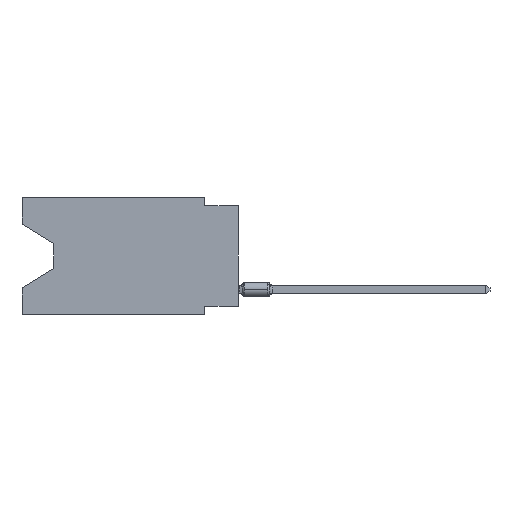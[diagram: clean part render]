
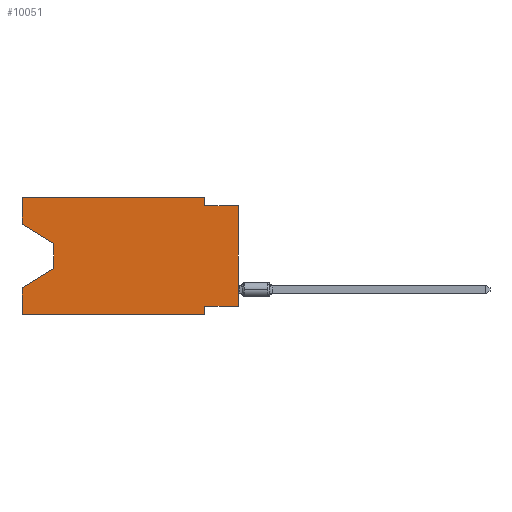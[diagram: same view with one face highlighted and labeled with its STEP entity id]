
A CAD part, left-side view. The second image highlights one B-rep face of the part: STEP entity #10051.
In plain terms, the highlighted planar face has unit normal (-1, 0, 0).
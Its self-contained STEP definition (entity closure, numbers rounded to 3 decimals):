
#285 = VERTEX_POINT ( 'NONE', #27186 ) ;
#914 = EDGE_CURVE ( 'NONE', #20251, #285, #4127, .T. ) ;
#1156 = EDGE_CURVE ( 'NONE', #26444, #12205, #14999, .T. ) ;
#1359 = ORIENTED_EDGE ( 'NONE', *, *, #14891, .F. ) ;
#1367 = CARTESIAN_POINT ( 'NONE',  ( 0., 0., -8.255 ) ) ;
#1900 = LINE ( 'NONE', #19036, #32785 ) ;
#2219 = DIRECTION ( 'NONE',  ( 0., 0.855, -0.519 ) ) ;
#2272 = VERTEX_POINT ( 'NONE', #8309 ) ;
#2441 = EDGE_CURVE ( 'NONE', #15579, #12205, #24383, .T. ) ;
#2508 = VERTEX_POINT ( 'NONE', #16016 ) ;
#3101 = VECTOR ( 'NONE', #3496, 1000. ) ;
#3142 = LINE ( 'NONE', #5683, #3101 ) ;
#3309 = DIRECTION ( 'NONE',  ( 1., 0., 0. ) ) ;
#3443 = VECTOR ( 'NONE', #9934, 1000. ) ;
#3496 = DIRECTION ( 'NONE',  ( 0., 0., 1. ) ) ;
#4127 = LINE ( 'NONE', #6864, #36004 ) ;
#4473 = DIRECTION ( 'NONE',  ( 0., -0.855, -0.519 ) ) ;
#4823 = VECTOR ( 'NONE', #21709, 1000. ) ;
#5070 = EDGE_LOOP ( 'NONE', ( #5786, #25630, #13512, #14981, #6533, #34944, #1359, #22528, #35115, #5859, #28084, #8815 ) ) ;
#5099 = VERTEX_POINT ( 'NONE', #5734 ) ;
#5683 = CARTESIAN_POINT ( 'NONE',  ( 0., 16.383, 0. ) ) ;
#5734 = CARTESIAN_POINT ( 'NONE',  ( 0., 16.383, -6.852 ) ) ;
#5786 = ORIENTED_EDGE ( 'NONE', *, *, #914, .T. ) ;
#5859 = ORIENTED_EDGE ( 'NONE', *, *, #7292, .F. ) ;
#5867 = PLANE ( 'NONE',  #7014 ) ;
#6010 = CARTESIAN_POINT ( 'NONE',  ( 0., 16.383, -8.89 ) ) ;
#6533 = ORIENTED_EDGE ( 'NONE', *, *, #31636, .T. ) ;
#6864 = CARTESIAN_POINT ( 'NONE',  ( 0., 16.383, -2.038 ) ) ;
#6902 = VECTOR ( 'NONE', #27831, 1000. ) ;
#7014 = AXIS2_PLACEMENT_3D ( 'NONE', #23020, #3309, #33968 ) ;
#7076 = CARTESIAN_POINT ( 'NONE',  ( 0., 13.97, -3.505 ) ) ;
#7292 = EDGE_CURVE ( 'NONE', #34059, #15579, #24285, .T. ) ;
#8011 = CARTESIAN_POINT ( 'NONE',  ( 0., 16.383, -8.89 ) ) ;
#8207 = VERTEX_POINT ( 'NONE', #30548 ) ;
#8309 = CARTESIAN_POINT ( 'NONE',  ( 0., 2.54, -8.89 ) ) ;
#8815 = ORIENTED_EDGE ( 'NONE', *, *, #31405, .F. ) ;
#9934 = DIRECTION ( 'NONE',  ( 0., 1., 0. ) ) ;
#9997 = LINE ( 'NONE', #7076, #15230 ) ;
#10051 = ADVANCED_FACE ( 'NONE', ( #17003 ), #5867, .F. ) ;
#10300 = DIRECTION ( 'NONE',  ( 0., 0., 1. ) ) ;
#11858 = VECTOR ( 'NONE', #2219, 1000. ) ;
#12205 = VERTEX_POINT ( 'NONE', #23962 ) ;
#13457 = DIRECTION ( 'NONE',  ( 0., -1., 0. ) ) ;
#13499 = LINE ( 'NONE', #8011, #4823 ) ;
#13512 = ORIENTED_EDGE ( 'NONE', *, *, #31322, .T. ) ;
#14691 = EDGE_CURVE ( 'NONE', #28630, #34059, #16705, .T. ) ;
#14891 = EDGE_CURVE ( 'NONE', #26444, #2508, #26363, .T. ) ;
#14909 = DIRECTION ( 'NONE',  ( 0., 0., -1. ) ) ;
#14981 = ORIENTED_EDGE ( 'NONE', *, *, #30806, .F. ) ;
#14999 = LINE ( 'NONE', #23205, #31960 ) ;
#15230 = VECTOR ( 'NONE', #23147, 1000. ) ;
#15334 = VECTOR ( 'NONE', #13457, 1000. ) ;
#15579 = VERTEX_POINT ( 'NONE', #20095 ) ;
#16016 = CARTESIAN_POINT ( 'NONE',  ( 0., 2.54, -8.255 ) ) ;
#16101 = CARTESIAN_POINT ( 'NONE',  ( 0., 16.383, 0. ) ) ;
#16273 = CARTESIAN_POINT ( 'NONE',  ( 0., 13.97, -5.385 ) ) ;
#16705 = LINE ( 'NONE', #32946, #6902 ) ;
#17003 = FACE_OUTER_BOUND ( 'NONE', #5070, .T. ) ;
#17646 = CARTESIAN_POINT ( 'NONE',  ( 0., 2.54, -8.89 ) ) ;
#18054 = CARTESIAN_POINT ( 'NONE',  ( 0., 16.383, -2.038 ) ) ;
#19036 = CARTESIAN_POINT ( 'NONE',  ( 0., 16.383, 0. ) ) ;
#20095 = CARTESIAN_POINT ( 'NONE',  ( 0., 2.54, -0.635 ) ) ;
#20251 = VERTEX_POINT ( 'NONE', #18054 ) ;
#20941 = CARTESIAN_POINT ( 'NONE',  ( 0., 0., -8.255 ) ) ;
#21709 = DIRECTION ( 'NONE',  ( 0., -1., 0. ) ) ;
#22205 = CARTESIAN_POINT ( 'NONE',  ( 0., 0., -0.635 ) ) ;
#22528 = ORIENTED_EDGE ( 'NONE', *, *, #1156, .T. ) ;
#23020 = CARTESIAN_POINT ( 'NONE',  ( 0., 16.383, 0. ) ) ;
#23147 = DIRECTION ( 'NONE',  ( 0., 0., -1. ) ) ;
#23205 = CARTESIAN_POINT ( 'NONE',  ( 0., 0., 0. ) ) ;
#23962 = CARTESIAN_POINT ( 'NONE',  ( 0., 0., -0.635 ) ) ;
#24285 = LINE ( 'NONE', #24470, #34152 ) ;
#24383 = LINE ( 'NONE', #22205, #15334 ) ;
#24470 = CARTESIAN_POINT ( 'NONE',  ( 0., 2.54, 0. ) ) ;
#25630 = ORIENTED_EDGE ( 'NONE', *, *, #26337, .T. ) ;
#25877 = VECTOR ( 'NONE', #14909, 1000. ) ;
#26220 = VERTEX_POINT ( 'NONE', #6010 ) ;
#26337 = EDGE_CURVE ( 'NONE', #285, #8207, #9997, .T. ) ;
#26363 = LINE ( 'NONE', #1367, #3443 ) ;
#26444 = VERTEX_POINT ( 'NONE', #20941 ) ;
#27186 = CARTESIAN_POINT ( 'NONE',  ( 0., 13.97, -3.505 ) ) ;
#27211 = LINE ( 'NONE', #16273, #11858 ) ;
#27831 = DIRECTION ( 'NONE',  ( 0., -1., 0. ) ) ;
#28084 = ORIENTED_EDGE ( 'NONE', *, *, #14691, .F. ) ;
#28630 = VERTEX_POINT ( 'NONE', #16101 ) ;
#29112 = LINE ( 'NONE', #17646, #25877 ) ;
#30548 = CARTESIAN_POINT ( 'NONE',  ( 0., 13.97, -5.385 ) ) ;
#30806 = EDGE_CURVE ( 'NONE', #26220, #5099, #1900, .T. ) ;
#31322 = EDGE_CURVE ( 'NONE', #8207, #5099, #27211, .T. ) ;
#31405 = EDGE_CURVE ( 'NONE', #20251, #28630, #3142, .T. ) ;
#31636 = EDGE_CURVE ( 'NONE', #26220, #2272, #13499, .T. ) ;
#31777 = DIRECTION ( 'NONE',  ( 0., 0., 1. ) ) ;
#31960 = VECTOR ( 'NONE', #31777, 1000. ) ;
#32302 = EDGE_CURVE ( 'NONE', #2508, #2272, #29112, .T. ) ;
#32785 = VECTOR ( 'NONE', #10300, 1000. ) ;
#32946 = CARTESIAN_POINT ( 'NONE',  ( 0., 16.383, 0. ) ) ;
#33205 = CARTESIAN_POINT ( 'NONE',  ( 0., 2.54, 0. ) ) ;
#33968 = DIRECTION ( 'NONE',  ( 0., 0., -1. ) ) ;
#34059 = VERTEX_POINT ( 'NONE', #33205 ) ;
#34152 = VECTOR ( 'NONE', #35421, 1000. ) ;
#34944 = ORIENTED_EDGE ( 'NONE', *, *, #32302, .F. ) ;
#35115 = ORIENTED_EDGE ( 'NONE', *, *, #2441, .F. ) ;
#35421 = DIRECTION ( 'NONE',  ( 0., 0., -1. ) ) ;
#36004 = VECTOR ( 'NONE', #4473, 1000. ) ;
